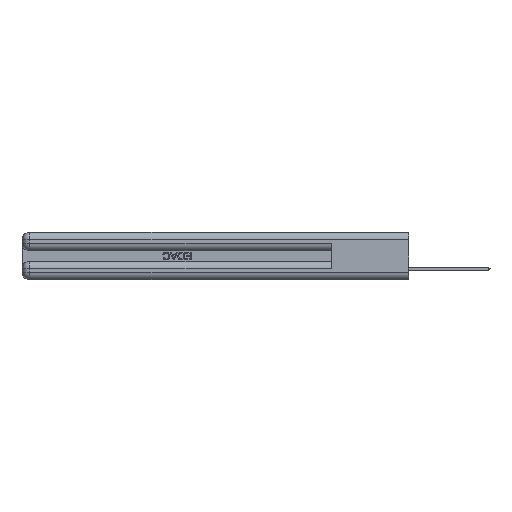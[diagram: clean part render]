
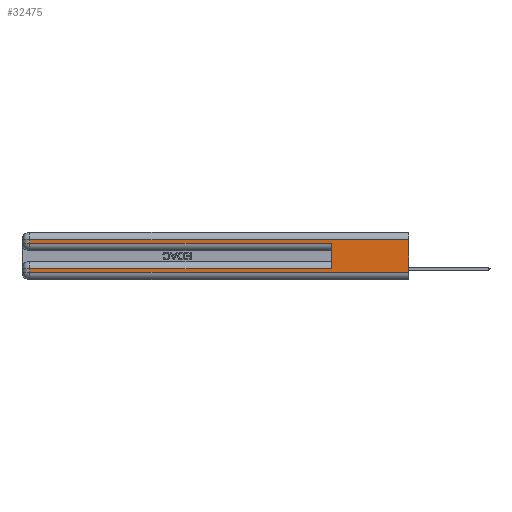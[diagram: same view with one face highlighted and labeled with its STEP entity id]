
A CAD part, left-side view. The second image highlights one B-rep face of the part: STEP entity #32475.
In plain terms, the highlighted planar face has unit normal (-1, 0, 0).
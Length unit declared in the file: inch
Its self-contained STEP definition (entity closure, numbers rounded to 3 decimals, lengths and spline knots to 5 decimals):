
#558 = FACE_OUTER_BOUND ( 'NONE', #3704, .T. ) ;
#1070 = DIRECTION ( 'NONE',  ( 0., -1., 0. ) ) ;
#1523 = DIRECTION ( 'NONE',  ( 0., 0., -1. ) ) ;
#2304 = CARTESIAN_POINT ( 'NONE',  ( 0., 0., 0.31 ) ) ;
#3229 = ORIENTED_EDGE ( 'NONE', *, *, #33598, .T. ) ;
#3268 = DIRECTION ( 'NONE',  ( 0., 0., 1. ) ) ;
#3704 = EDGE_LOOP ( 'NONE', ( #12507, #20878, #17523, #3229, #10544, #32892, #13998, #38761 ) ) ;
#3797 = CARTESIAN_POINT ( 'NONE',  ( 0., 2.94, 0.37 ) ) ;
#4647 = VERTEX_POINT ( 'NONE', #37863 ) ;
#4768 = LINE ( 'NONE', #3797, #42039 ) ;
#6678 = DIRECTION ( 'NONE',  ( 0., 0., -1. ) ) ;
#6844 = CARTESIAN_POINT ( 'NONE',  ( 0., 0.6, 0.285 ) ) ;
#6954 = VECTOR ( 'NONE', #1523, 39.37008 ) ;
#7820 = VECTOR ( 'NONE', #37080, 39.37008 ) ;
#8276 = AXIS2_PLACEMENT_3D ( 'NONE', #27993, #31622, #6678 ) ;
#8422 = LINE ( 'NONE', #23833, #33847 ) ;
#8941 = LINE ( 'NONE', #33080, #44507 ) ;
#9844 = VERTEX_POINT ( 'NONE', #27215 ) ;
#9948 = PLANE ( 'NONE',  #8276 ) ;
#10544 = ORIENTED_EDGE ( 'NONE', *, *, #40108, .F. ) ;
#10874 = CARTESIAN_POINT ( 'NONE',  ( 0., 0.6, 0.145 ) ) ;
#10903 = CARTESIAN_POINT ( 'NONE',  ( 0., 2.94, 0.37 ) ) ;
#11953 = VECTOR ( 'NONE', #25472, 39.37008 ) ;
#12507 = ORIENTED_EDGE ( 'NONE', *, *, #27043, .F. ) ;
#13097 = DIRECTION ( 'NONE',  ( 0., 1., 0. ) ) ;
#13998 = ORIENTED_EDGE ( 'NONE', *, *, #20862, .T. ) ;
#15260 = VERTEX_POINT ( 'NONE', #41640 ) ;
#16910 = CARTESIAN_POINT ( 'NONE',  ( 0., 2.94, 0.085 ) ) ;
#17523 = ORIENTED_EDGE ( 'NONE', *, *, #27472, .T. ) ;
#18544 = CARTESIAN_POINT ( 'NONE',  ( 0., 2.94, 0.31 ) ) ;
#18947 = VERTEX_POINT ( 'NONE', #16910 ) ;
#19048 = LINE ( 'NONE', #2304, #33734 ) ;
#19558 = DIRECTION ( 'NONE',  ( 0., 0., -1. ) ) ;
#20862 = EDGE_CURVE ( 'NONE', #18947, #4647, #4768, .T. ) ;
#20878 = ORIENTED_EDGE ( 'NONE', *, *, #37678, .T. ) ;
#22221 = VERTEX_POINT ( 'NONE', #30426 ) ;
#23833 = CARTESIAN_POINT ( 'NONE',  ( 0., 0., 0.085 ) ) ;
#24472 = DIRECTION ( 'NONE',  ( 0., 1., 0. ) ) ;
#25472 = DIRECTION ( 'NONE',  ( 0., 0., -1. ) ) ;
#26763 = VECTOR ( 'NONE', #3268, 39.37008 ) ;
#26901 = VERTEX_POINT ( 'NONE', #18544 ) ;
#27043 = EDGE_CURVE ( 'NONE', #9844, #15260, #32895, .T. ) ;
#27215 = CARTESIAN_POINT ( 'NONE',  ( 0., 0., 0.31 ) ) ;
#27472 = EDGE_CURVE ( 'NONE', #26901, #43969, #31776, .T. ) ;
#27993 = CARTESIAN_POINT ( 'NONE',  ( 0., 0., 0.37 ) ) ;
#29858 = CARTESIAN_POINT ( 'NONE',  ( 0., 0., 0.37 ) ) ;
#29972 = CARTESIAN_POINT ( 'NONE',  ( 0., 2.94, 0.285 ) ) ;
#30141 = LINE ( 'NONE', #10874, #26763 ) ;
#30426 = CARTESIAN_POINT ( 'NONE',  ( 0., 0.6, 0.085 ) ) ;
#31622 = DIRECTION ( 'NONE',  ( 1., 0., 0. ) ) ;
#31776 = LINE ( 'NONE', #10903, #11953 ) ;
#31926 = VERTEX_POINT ( 'NONE', #6844 ) ;
#32475 = ADVANCED_FACE ( 'NONE', ( #558 ), #9948, .F. ) ;
#32892 = ORIENTED_EDGE ( 'NONE', *, *, #33214, .T. ) ;
#32895 = LINE ( 'NONE', #29858, #6954 ) ;
#33080 = CARTESIAN_POINT ( 'NONE',  ( 0., 0., 0.06 ) ) ;
#33214 = EDGE_CURVE ( 'NONE', #22221, #18947, #8422, .T. ) ;
#33598 = EDGE_CURVE ( 'NONE', #43969, #31926, #40016, .T. ) ;
#33734 = VECTOR ( 'NONE', #13097, 39.37008 ) ;
#33847 = VECTOR ( 'NONE', #24472, 39.37008 ) ;
#34154 = EDGE_CURVE ( 'NONE', #4647, #15260, #8941, .T. ) ;
#37080 = DIRECTION ( 'NONE',  ( 0., -1., 0. ) ) ;
#37678 = EDGE_CURVE ( 'NONE', #9844, #26901, #19048, .T. ) ;
#37863 = CARTESIAN_POINT ( 'NONE',  ( 0., 2.94, 0.06 ) ) ;
#38761 = ORIENTED_EDGE ( 'NONE', *, *, #34154, .T. ) ;
#40016 = LINE ( 'NONE', #44036, #7820 ) ;
#40108 = EDGE_CURVE ( 'NONE', #22221, #31926, #30141, .T. ) ;
#41640 = CARTESIAN_POINT ( 'NONE',  ( 0., 0., 0.06 ) ) ;
#42039 = VECTOR ( 'NONE', #19558, 39.37008 ) ;
#43969 = VERTEX_POINT ( 'NONE', #29972 ) ;
#44036 = CARTESIAN_POINT ( 'NONE',  ( 0., 0., 0.285 ) ) ;
#44507 = VECTOR ( 'NONE', #1070, 39.37008 ) ;
